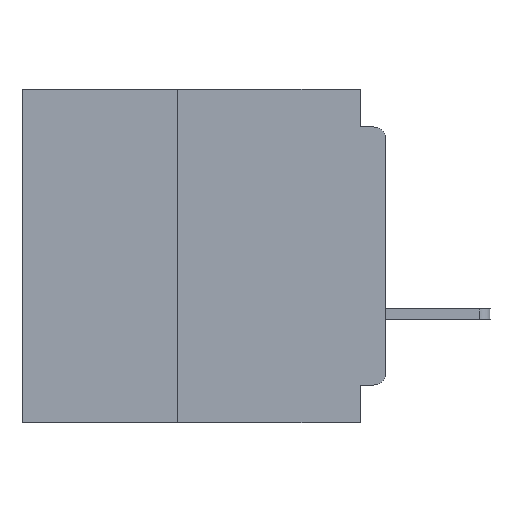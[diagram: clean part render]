
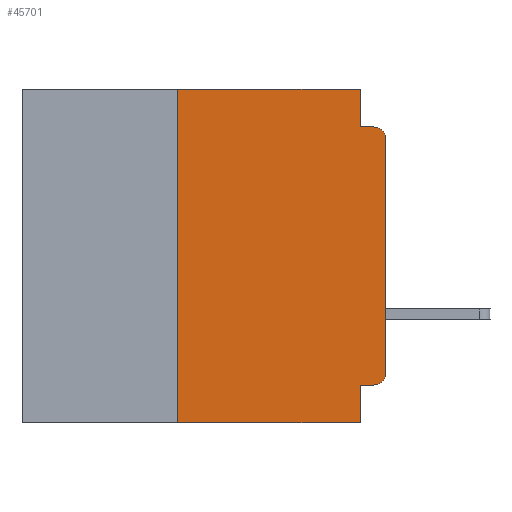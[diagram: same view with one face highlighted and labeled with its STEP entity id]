
A CAD part, left-side view. The second image highlights one B-rep face of the part: STEP entity #45701.
In plain terms, the highlighted planar face has unit normal (-1, 0, 0).
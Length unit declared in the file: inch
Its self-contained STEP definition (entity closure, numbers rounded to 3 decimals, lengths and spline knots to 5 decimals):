
#346 = CIRCLE ( 'NONE', #22076, 0.015 ) ;
#1819 = CARTESIAN_POINT ( 'NONE',  ( 0., 0.031, -0.355 ) ) ;
#3554 = ORIENTED_EDGE ( 'NONE', *, *, #15290, .F. ) ;
#3788 = CARTESIAN_POINT ( 'NONE',  ( 0., 0.25, -0.4 ) ) ;
#3875 = EDGE_CURVE ( 'NONE', #28425, #44068, #6781, .T. ) ;
#4646 = VERTEX_POINT ( 'NONE', #1819 ) ;
#5366 = DIRECTION ( 'NONE',  ( 0., 1., 0. ) ) ;
#5670 = EDGE_CURVE ( 'NONE', #18187, #55015, #42670, .T. ) ;
#5813 = VERTEX_POINT ( 'NONE', #11308 ) ;
#6505 = VECTOR ( 'NONE', #8568, 39.37008 ) ;
#6687 = CARTESIAN_POINT ( 'NONE',  ( 0., 0., -0.045 ) ) ;
#6781 = LINE ( 'NONE', #24976, #40437 ) ;
#6861 = VECTOR ( 'NONE', #5366, 39.37008 ) ;
#7228 = ORIENTED_EDGE ( 'NONE', *, *, #50959, .T. ) ;
#8199 = VECTOR ( 'NONE', #13087, 39.37008 ) ;
#8568 = DIRECTION ( 'NONE',  ( 0., 0., -1. ) ) ;
#8765 = CARTESIAN_POINT ( 'NONE',  ( 0., 0.031, -0.4 ) ) ;
#9260 = EDGE_CURVE ( 'NONE', #31351, #53225, #53647, .T. ) ;
#9817 = CARTESIAN_POINT ( 'NONE',  ( 0., 0., -0.355 ) ) ;
#10440 = VECTOR ( 'NONE', #18842, 39.37008 ) ;
#11035 = DIRECTION ( 'NONE',  ( -1., 0., 0. ) ) ;
#11154 = DIRECTION ( 'NONE',  ( 0., -1., 0. ) ) ;
#11290 = CARTESIAN_POINT ( 'NONE',  ( 0., 0.031, 0. ) ) ;
#11308 = CARTESIAN_POINT ( 'NONE',  ( 0., 0.031, -0.4 ) ) ;
#13087 = DIRECTION ( 'NONE',  ( 0., -1., 0. ) ) ;
#13835 = EDGE_CURVE ( 'NONE', #55015, #50791, #45739, .T. ) ;
#13869 = ORIENTED_EDGE ( 'NONE', *, *, #45728, .T. ) ;
#13949 = ORIENTED_EDGE ( 'NONE', *, *, #13835, .F. ) ;
#15290 = EDGE_CURVE ( 'NONE', #4646, #5813, #28708, .T. ) ;
#15526 = DIRECTION ( 'NONE',  ( 1., 0., 0. ) ) ;
#16420 = CARTESIAN_POINT ( 'NONE',  ( 0., 0.031, 0. ) ) ;
#18187 = VERTEX_POINT ( 'NONE', #3788 ) ;
#18842 = DIRECTION ( 'NONE',  ( 0., 0., 1. ) ) ;
#18898 = CARTESIAN_POINT ( 'NONE',  ( 0., 0.25, -0.4 ) ) ;
#20597 = CARTESIAN_POINT ( 'NONE',  ( 0., 0.015, -0.355 ) ) ;
#20870 = DIRECTION ( 'NONE',  ( 0., 0., 1. ) ) ;
#22076 = AXIS2_PLACEMENT_3D ( 'NONE', #37375, #11035, #41707 ) ;
#24233 = PLANE ( 'NONE',  #51048 ) ;
#24321 = EDGE_CURVE ( 'NONE', #47659, #4646, #30391, .T. ) ;
#24635 = CARTESIAN_POINT ( 'NONE',  ( 0., 0.015, -0.06 ) ) ;
#24976 = CARTESIAN_POINT ( 'NONE',  ( 0., 0., 0. ) ) ;
#26872 = ORIENTED_EDGE ( 'NONE', *, *, #39519, .T. ) ;
#28425 = VERTEX_POINT ( 'NONE', #39918 ) ;
#28698 = CARTESIAN_POINT ( 'NONE',  ( 0., 0.437, 0. ) ) ;
#28708 = LINE ( 'NONE', #8765, #6505 ) ;
#29062 = DIRECTION ( 'NONE',  ( 0., 0., -1. ) ) ;
#30391 = LINE ( 'NONE', #9817, #6861 ) ;
#31351 = VERTEX_POINT ( 'NONE', #45639 ) ;
#31490 = FACE_OUTER_BOUND ( 'NONE', #53665, .T. ) ;
#32034 = VECTOR ( 'NONE', #11154, 39.37008 ) ;
#32935 = EDGE_CURVE ( 'NONE', #50791, #31351, #42767, .T. ) ;
#34271 = VECTOR ( 'NONE', #55947, 39.37008 ) ;
#34648 = ORIENTED_EDGE ( 'NONE', *, *, #5670, .F. ) ;
#35022 = CARTESIAN_POINT ( 'NONE',  ( 0., 0.437, -0.4 ) ) ;
#36894 = ORIENTED_EDGE ( 'NONE', *, *, #3875, .T. ) ;
#37375 = CARTESIAN_POINT ( 'NONE',  ( 0., 0.015, -0.34 ) ) ;
#39519 = EDGE_CURVE ( 'NONE', #47659, #28425, #346, .T. ) ;
#39918 = CARTESIAN_POINT ( 'NONE',  ( 0., 0., -0.34 ) ) ;
#40437 = VECTOR ( 'NONE', #20870, 39.37008 ) ;
#41586 = CIRCLE ( 'NONE', #53946, 0.015 ) ;
#41707 = DIRECTION ( 'NONE',  ( 0., 0., -1. ) ) ;
#42670 = LINE ( 'NONE', #18898, #10440 ) ;
#42767 = LINE ( 'NONE', #11290, #55608 ) ;
#43757 = CARTESIAN_POINT ( 'NONE',  ( 0., 0.015, -0.045 ) ) ;
#44068 = VERTEX_POINT ( 'NONE', #46420 ) ;
#45639 = CARTESIAN_POINT ( 'NONE',  ( 0., 0.031, -0.045 ) ) ;
#45701 = ADVANCED_FACE ( 'NONE', ( #31490 ), #24233, .F. ) ;
#45728 = EDGE_CURVE ( 'NONE', #44068, #53225, #41586, .T. ) ;
#45739 = LINE ( 'NONE', #47261, #34271 ) ;
#46017 = CARTESIAN_POINT ( 'NONE',  ( 0., 0.25, 0. ) ) ;
#46034 = DIRECTION ( 'NONE',  ( 0., 0., -1. ) ) ;
#46264 = DIRECTION ( 'NONE',  ( 0., 0., -1. ) ) ;
#46393 = ORIENTED_EDGE ( 'NONE', *, *, #32935, .F. ) ;
#46420 = CARTESIAN_POINT ( 'NONE',  ( 0., 0., -0.06 ) ) ;
#47261 = CARTESIAN_POINT ( 'NONE',  ( 0., 0.437, 0. ) ) ;
#47568 = ORIENTED_EDGE ( 'NONE', *, *, #9260, .F. ) ;
#47659 = VERTEX_POINT ( 'NONE', #20597 ) ;
#50791 = VERTEX_POINT ( 'NONE', #16420 ) ;
#50959 = EDGE_CURVE ( 'NONE', #18187, #5813, #51997, .T. ) ;
#51048 = AXIS2_PLACEMENT_3D ( 'NONE', #28698, #15526, #46034 ) ;
#51997 = LINE ( 'NONE', #35022, #8199 ) ;
#53225 = VERTEX_POINT ( 'NONE', #43757 ) ;
#53647 = LINE ( 'NONE', #6687, #32034 ) ;
#53665 = EDGE_LOOP ( 'NONE', ( #36894, #13869, #47568, #46393, #13949, #34648, #7228, #3554, #56745, #26872 ) ) ;
#53946 = AXIS2_PLACEMENT_3D ( 'NONE', #24635, #54932, #29062 ) ;
#54932 = DIRECTION ( 'NONE',  ( -1., 0., 0. ) ) ;
#55015 = VERTEX_POINT ( 'NONE', #46017 ) ;
#55608 = VECTOR ( 'NONE', #46264, 39.37008 ) ;
#55947 = DIRECTION ( 'NONE',  ( 0., -1., 0. ) ) ;
#56745 = ORIENTED_EDGE ( 'NONE', *, *, #24321, .F. ) ;
